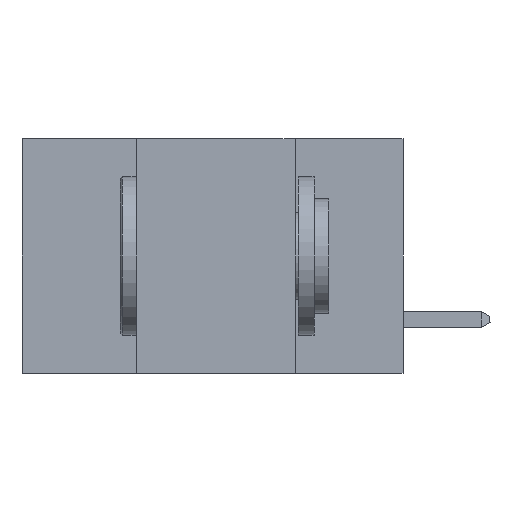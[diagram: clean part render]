
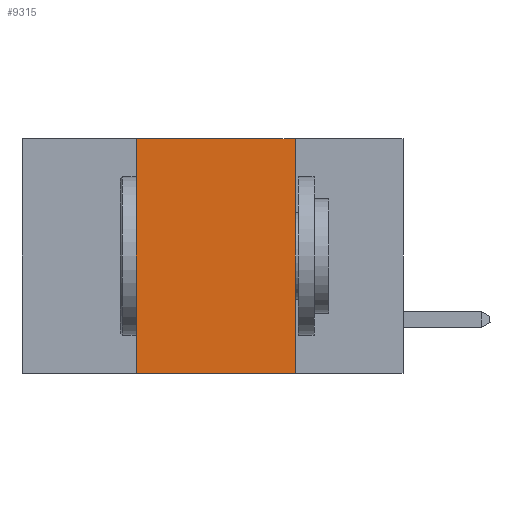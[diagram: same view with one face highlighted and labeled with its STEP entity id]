
A CAD part, left-side view. The second image highlights one B-rep face of the part: STEP entity #9315.
In plain terms, the highlighted planar face has unit normal (-1, 0, 0).
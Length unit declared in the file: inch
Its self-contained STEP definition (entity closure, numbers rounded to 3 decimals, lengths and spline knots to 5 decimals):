
#564 = DIRECTION ( 'NONE',  ( 1., 0., 0. ) ) ;
#2587 = LINE ( 'NONE', #7792, #20839 ) ;
#5262 = EDGE_CURVE ( 'NONE', #22399, #10735, #28163, .T. ) ;
#6867 = VECTOR ( 'NONE', #10333, 39.37008 ) ;
#7294 = AXIS2_PLACEMENT_3D ( 'NONE', #16524, #564, #11114 ) ;
#7595 = ORIENTED_EDGE ( 'NONE', *, *, #5262, .T. ) ;
#7792 = CARTESIAN_POINT ( 'NONE',  ( 0., 0.17, 0. ) ) ;
#8420 = CARTESIAN_POINT ( 'NONE',  ( 0., 0.6, 0. ) ) ;
#9315 = ADVANCED_FACE ( 'NONE', ( #25667 ), #24015, .F. ) ;
#9411 = ORIENTED_EDGE ( 'NONE', *, *, #27588, .F. ) ;
#9814 = VECTOR ( 'NONE', #32578, 39.37008 ) ;
#10333 = DIRECTION ( 'NONE',  ( 0., 0., 1. ) ) ;
#10735 = VERTEX_POINT ( 'NONE', #32639 ) ;
#11114 = DIRECTION ( 'NONE',  ( 0., 0., -1. ) ) ;
#11340 = DIRECTION ( 'NONE',  ( 0., -1., 0. ) ) ;
#12199 = VECTOR ( 'NONE', #11340, 39.37008 ) ;
#12404 = EDGE_LOOP ( 'NONE', ( #25102, #30249, #9411, #7595 ) ) ;
#14359 = VERTEX_POINT ( 'NONE', #16643 ) ;
#16029 = EDGE_CURVE ( 'NONE', #16946, #14359, #17385, .T. ) ;
#16524 = CARTESIAN_POINT ( 'NONE',  ( 0., 0.6, 0. ) ) ;
#16643 = CARTESIAN_POINT ( 'NONE',  ( 0., 0.17, 0. ) ) ;
#16946 = VERTEX_POINT ( 'NONE', #27072 ) ;
#16993 = CARTESIAN_POINT ( 'NONE',  ( 0., 0.6, -0.37 ) ) ;
#17385 = LINE ( 'NONE', #8420, #12199 ) ;
#20839 = VECTOR ( 'NONE', #23161, 39.37008 ) ;
#22399 = VERTEX_POINT ( 'NONE', #30315 ) ;
#23161 = DIRECTION ( 'NONE',  ( 0., 0., -1. ) ) ;
#24015 = PLANE ( 'NONE',  #7294 ) ;
#25102 = ORIENTED_EDGE ( 'NONE', *, *, #26253, .F. ) ;
#25667 = FACE_OUTER_BOUND ( 'NONE', #12404, .T. ) ;
#26253 = EDGE_CURVE ( 'NONE', #14359, #10735, #2587, .T. ) ;
#27072 = CARTESIAN_POINT ( 'NONE',  ( 0., 0.42, 0. ) ) ;
#27588 = EDGE_CURVE ( 'NONE', #22399, #16946, #32033, .T. ) ;
#28163 = LINE ( 'NONE', #16993, #9814 ) ;
#28180 = CARTESIAN_POINT ( 'NONE',  ( 0., 0.42, 0. ) ) ;
#30249 = ORIENTED_EDGE ( 'NONE', *, *, #16029, .F. ) ;
#30315 = CARTESIAN_POINT ( 'NONE',  ( 0., 0.42, -0.37 ) ) ;
#32033 = LINE ( 'NONE', #28180, #6867 ) ;
#32578 = DIRECTION ( 'NONE',  ( 0., -1., 0. ) ) ;
#32639 = CARTESIAN_POINT ( 'NONE',  ( 0., 0.17, -0.37 ) ) ;
